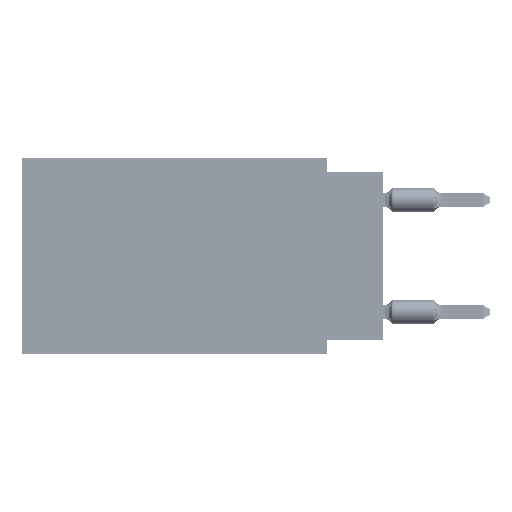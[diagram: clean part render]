
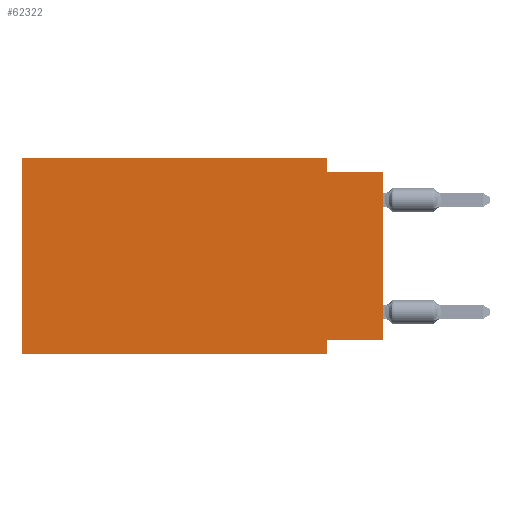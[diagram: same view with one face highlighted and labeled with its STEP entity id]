
A CAD part, left-side view. The second image highlights one B-rep face of the part: STEP entity #62322.
In plain terms, the highlighted planar face has unit normal (-1, 0, 0).
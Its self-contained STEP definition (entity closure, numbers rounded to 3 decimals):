
#4519 = EDGE_CURVE ( 'NONE', #102592, #21130, #50829, .T. ) ;
#5194 = VERTEX_POINT ( 'NONE', #83279 ) ;
#8049 = VECTOR ( 'NONE', #86117, 1000. ) ;
#9995 = EDGE_CURVE ( 'NONE', #5194, #21961, #15395, .T. ) ;
#11188 = EDGE_CURVE ( 'NONE', #45598, #102592, #90799, .T. ) ;
#11418 = DIRECTION ( 'NONE',  ( 0., 0., -1. ) ) ;
#11683 = DIRECTION ( 'NONE',  ( 0., 1., 0. ) ) ;
#11737 = ORIENTED_EDGE ( 'NONE', *, *, #79895, .F. ) ;
#12010 = EDGE_CURVE ( 'NONE', #12561, #21961, #47287, .T. ) ;
#12561 = VERTEX_POINT ( 'NONE', #47560 ) ;
#12848 = CARTESIAN_POINT ( 'NONE',  ( 0., 16.383, 0. ) ) ;
#13947 = DIRECTION ( 'NONE',  ( 0., 0., -1. ) ) ;
#14821 = CARTESIAN_POINT ( 'NONE',  ( 0., 16.383, 0. ) ) ;
#15395 = LINE ( 'NONE', #100747, #48693 ) ;
#17068 = ORIENTED_EDGE ( 'NONE', *, *, #79409, .F. ) ;
#18944 = LINE ( 'NONE', #19503, #54781 ) ;
#19503 = CARTESIAN_POINT ( 'NONE',  ( 0., 16.383, -8.89 ) ) ;
#21130 = VERTEX_POINT ( 'NONE', #89544 ) ;
#21961 = VERTEX_POINT ( 'NONE', #46035 ) ;
#22671 = ORIENTED_EDGE ( 'NONE', *, *, #4519, .F. ) ;
#25014 = DIRECTION ( 'NONE',  ( 0., 0., -1. ) ) ;
#25236 = CARTESIAN_POINT ( 'NONE',  ( 0., 16.383, 0. ) ) ;
#27249 = VECTOR ( 'NONE', #13947, 1000. ) ;
#27984 = ORIENTED_EDGE ( 'NONE', *, *, #12010, .T. ) ;
#31470 = ORIENTED_EDGE ( 'NONE', *, *, #11188, .F. ) ;
#33869 = VERTEX_POINT ( 'NONE', #83396 ) ;
#39298 = CARTESIAN_POINT ( 'NONE',  ( 0., 0., 0. ) ) ;
#45598 = VERTEX_POINT ( 'NONE', #81523 ) ;
#46035 = CARTESIAN_POINT ( 'NONE',  ( 0., 0., -0.635 ) ) ;
#46598 = EDGE_CURVE ( 'NONE', #97239, #33869, #48068, .T. ) ;
#47287 = LINE ( 'NONE', #39298, #78417 ) ;
#47560 = CARTESIAN_POINT ( 'NONE',  ( 0., 0., -8.255 ) ) ;
#47833 = DIRECTION ( 'NONE',  ( 0., -1., 0. ) ) ;
#48068 = LINE ( 'NONE', #82794, #27249 ) ;
#48100 = ORIENTED_EDGE ( 'NONE', *, *, #46598, .F. ) ;
#48693 = VECTOR ( 'NONE', #47833, 1000. ) ;
#50829 = LINE ( 'NONE', #25236, #8049 ) ;
#53775 = CARTESIAN_POINT ( 'NONE',  ( 0., 0., -8.255 ) ) ;
#54781 = VECTOR ( 'NONE', #79830, 1000. ) ;
#62322 = ADVANCED_FACE ( 'NONE', ( #105199 ), #103548, .F. ) ;
#71950 = AXIS2_PLACEMENT_3D ( 'NONE', #86464, #87564, #25014 ) ;
#73409 = LINE ( 'NONE', #97899, #106495 ) ;
#73711 = DIRECTION ( 'NONE',  ( 0., 0., 1. ) ) ;
#78417 = VECTOR ( 'NONE', #81999, 1000. ) ;
#79409 = EDGE_CURVE ( 'NONE', #12561, #97239, #98176, .T. ) ;
#79759 = ORIENTED_EDGE ( 'NONE', *, *, #9995, .F. ) ;
#79830 = DIRECTION ( 'NONE',  ( 0., -1., 0. ) ) ;
#79895 = EDGE_CURVE ( 'NONE', #21130, #5194, #73409, .T. ) ;
#81523 = CARTESIAN_POINT ( 'NONE',  ( 0., 16.383, -8.89 ) ) ;
#81999 = DIRECTION ( 'NONE',  ( 0., 0., 1. ) ) ;
#82794 = CARTESIAN_POINT ( 'NONE',  ( 0., 2.54, -8.89 ) ) ;
#83279 = CARTESIAN_POINT ( 'NONE',  ( 0., 2.54, -0.635 ) ) ;
#83396 = CARTESIAN_POINT ( 'NONE',  ( 0., 2.54, -8.89 ) ) ;
#86117 = DIRECTION ( 'NONE',  ( 0., -1., 0. ) ) ;
#86464 = CARTESIAN_POINT ( 'NONE',  ( 0., 16.383, 0. ) ) ;
#87564 = DIRECTION ( 'NONE',  ( 1., 0., 0. ) ) ;
#89491 = EDGE_CURVE ( 'NONE', #45598, #33869, #18944, .T. ) ;
#89544 = CARTESIAN_POINT ( 'NONE',  ( 0., 2.54, 0. ) ) ;
#90799 = LINE ( 'NONE', #12848, #96338 ) ;
#92317 = VECTOR ( 'NONE', #11683, 1000. ) ;
#96338 = VECTOR ( 'NONE', #73711, 1000. ) ;
#97239 = VERTEX_POINT ( 'NONE', #101066 ) ;
#97899 = CARTESIAN_POINT ( 'NONE',  ( 0., 2.54, 0. ) ) ;
#98176 = LINE ( 'NONE', #53775, #92317 ) ;
#100747 = CARTESIAN_POINT ( 'NONE',  ( 0., 0., -0.635 ) ) ;
#101066 = CARTESIAN_POINT ( 'NONE',  ( 0., 2.54, -8.255 ) ) ;
#102592 = VERTEX_POINT ( 'NONE', #14821 ) ;
#102895 = ORIENTED_EDGE ( 'NONE', *, *, #89491, .T. ) ;
#103548 = PLANE ( 'NONE',  #71950 ) ;
#105199 = FACE_OUTER_BOUND ( 'NONE', #105572, .T. ) ;
#105572 = EDGE_LOOP ( 'NONE', ( #27984, #79759, #11737, #22671, #31470, #102895, #48100, #17068 ) ) ;
#106495 = VECTOR ( 'NONE', #11418, 1000. ) ;
